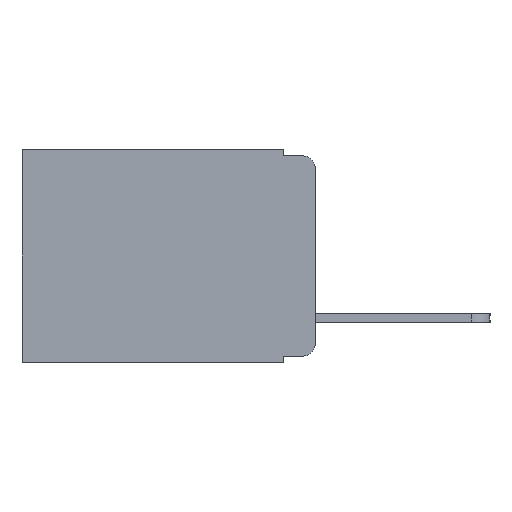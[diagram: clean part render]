
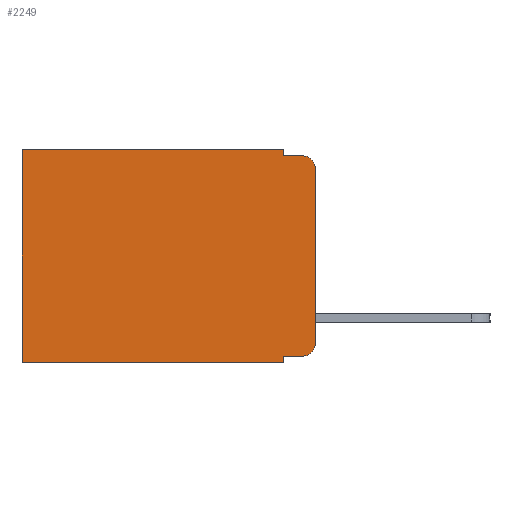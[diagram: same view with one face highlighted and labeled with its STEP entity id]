
A CAD part, left-side view. The second image highlights one B-rep face of the part: STEP entity #2249.
In plain terms, the highlighted planar face has unit normal (-1, 0, 0).
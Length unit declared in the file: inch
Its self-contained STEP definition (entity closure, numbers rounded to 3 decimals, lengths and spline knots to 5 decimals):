
#41 = CARTESIAN_POINT ( 'NONE',  ( 0.298, 0.473, 0. ) ) ;
#159 = DIRECTION ( 'NONE',  ( 0., 0., -1. ) ) ;
#184 = LINE ( 'NONE', #3766, #10985 ) ;
#445 = DIRECTION ( 'NONE',  ( 0., 1., 0. ) ) ;
#543 = ORIENTED_EDGE ( 'NONE', *, *, #4865, .F. ) ;
#1280 = CARTESIAN_POINT ( 'NONE',  ( 0.298, 0.051, -0.333 ) ) ;
#1439 = VECTOR ( 'NONE', #3045, 39.37008 ) ;
#1519 = LINE ( 'NONE', #2799, #8188 ) ;
#1610 = CARTESIAN_POINT ( 'NONE',  ( 0.298, 0.051, 0. ) ) ;
#1656 = AXIS2_PLACEMENT_3D ( 'NONE', #9635, #9394, #10530 ) ;
#1997 = ORIENTED_EDGE ( 'NONE', *, *, #7256, .F. ) ;
#2103 = CARTESIAN_POINT ( 'NONE',  ( 0.298, 0., -0.03 ) ) ;
#2249 = ADVANCED_FACE ( 'NONE', ( #2327 ), #7450, .F. ) ;
#2327 = FACE_OUTER_BOUND ( 'NONE', #2737, .T. ) ;
#2385 = VERTEX_POINT ( 'NONE', #4756 ) ;
#2593 = VERTEX_POINT ( 'NONE', #4092 ) ;
#2705 = VECTOR ( 'NONE', #5661, 39.37008 ) ;
#2737 = EDGE_LOOP ( 'NONE', ( #7662, #4558, #4544, #8062, #3162, #4737, #1997, #543, #10494, #10239 ) ) ;
#2799 = CARTESIAN_POINT ( 'NONE',  ( 0.298, 0., 0. ) ) ;
#2923 = DIRECTION ( 'NONE',  ( 0., 0., -1. ) ) ;
#2946 = CARTESIAN_POINT ( 'NONE',  ( 0.298, 0.473, 0. ) ) ;
#3045 = DIRECTION ( 'NONE',  ( 0., -1., 0. ) ) ;
#3051 = EDGE_CURVE ( 'NONE', #2385, #2593, #7707, .T. ) ;
#3162 = ORIENTED_EDGE ( 'NONE', *, *, #10858, .T. ) ;
#3249 = VECTOR ( 'NONE', #159, 39.37008 ) ;
#3407 = VECTOR ( 'NONE', #11004, 39.37008 ) ;
#3602 = AXIS2_PLACEMENT_3D ( 'NONE', #5839, #8775, #5685 ) ;
#3766 = CARTESIAN_POINT ( 'NONE',  ( 0.298, 0.051, 0. ) ) ;
#3966 = VERTEX_POINT ( 'NONE', #6133 ) ;
#3986 = VERTEX_POINT ( 'NONE', #1610 ) ;
#4092 = CARTESIAN_POINT ( 'NONE',  ( 0.298, 0., -0.313 ) ) ;
#4104 = VERTEX_POINT ( 'NONE', #2103 ) ;
#4249 = EDGE_CURVE ( 'NONE', #7365, #2385, #10185, .T. ) ;
#4544 = ORIENTED_EDGE ( 'NONE', *, *, #7107, .F. ) ;
#4558 = ORIENTED_EDGE ( 'NONE', *, *, #7637, .T. ) ;
#4737 = ORIENTED_EDGE ( 'NONE', *, *, #5451, .T. ) ;
#4756 = CARTESIAN_POINT ( 'NONE',  ( 0.298, 0.02, -0.333 ) ) ;
#4768 = CARTESIAN_POINT ( 'NONE',  ( 0.298, 0.051, -0.343 ) ) ;
#4865 = EDGE_CURVE ( 'NONE', #7365, #6795, #9928, .T. ) ;
#4984 = VERTEX_POINT ( 'NONE', #10301 ) ;
#5124 = CARTESIAN_POINT ( 'NONE',  ( 0.298, 0.02, -0.03 ) ) ;
#5451 = EDGE_CURVE ( 'NONE', #5745, #3966, #7301, .T. ) ;
#5661 = DIRECTION ( 'NONE',  ( 0., 0., -1. ) ) ;
#5685 = DIRECTION ( 'NONE',  ( 0., 0., -1. ) ) ;
#5745 = VERTEX_POINT ( 'NONE', #41 ) ;
#5839 = CARTESIAN_POINT ( 'NONE',  ( 0.298, 0., 0. ) ) ;
#5983 = DIRECTION ( 'NONE',  ( 0., 0., -1. ) ) ;
#6017 = EDGE_CURVE ( 'NONE', #3986, #4984, #184, .T. ) ;
#6046 = LINE ( 'NONE', #6265, #3407 ) ;
#6133 = CARTESIAN_POINT ( 'NONE',  ( 0.298, 0.473, -0.343 ) ) ;
#6265 = CARTESIAN_POINT ( 'NONE',  ( 0.298, 0., 0. ) ) ;
#6286 = CARTESIAN_POINT ( 'NONE',  ( 0.298, 0.051, 0. ) ) ;
#6609 = CARTESIAN_POINT ( 'NONE',  ( 0.298, 0.051, -0.333 ) ) ;
#6795 = VERTEX_POINT ( 'NONE', #4768 ) ;
#7107 = EDGE_CURVE ( 'NONE', #4984, #10355, #10242, .T. ) ;
#7256 = EDGE_CURVE ( 'NONE', #6795, #3966, #10835, .T. ) ;
#7301 = LINE ( 'NONE', #2946, #2705 ) ;
#7365 = VERTEX_POINT ( 'NONE', #1280 ) ;
#7450 = PLANE ( 'NONE',  #3602 ) ;
#7637 = EDGE_CURVE ( 'NONE', #4104, #10355, #9751, .T. ) ;
#7662 = ORIENTED_EDGE ( 'NONE', *, *, #10304, .F. ) ;
#7707 = CIRCLE ( 'NONE', #1656, 0.02 ) ;
#8061 = VECTOR ( 'NONE', #9763, 39.37008 ) ;
#8062 = ORIENTED_EDGE ( 'NONE', *, *, #6017, .F. ) ;
#8188 = VECTOR ( 'NONE', #9561, 39.37008 ) ;
#8421 = AXIS2_PLACEMENT_3D ( 'NONE', #5124, #10755, #5983 ) ;
#8756 = VECTOR ( 'NONE', #445, 39.37008 ) ;
#8775 = DIRECTION ( 'NONE',  ( 1., 0., 0. ) ) ;
#8828 = CARTESIAN_POINT ( 'NONE',  ( 0.298, 0.02, -0.01 ) ) ;
#9394 = DIRECTION ( 'NONE',  ( -1., 0., 0. ) ) ;
#9561 = DIRECTION ( 'NONE',  ( 0., 0., -1. ) ) ;
#9635 = CARTESIAN_POINT ( 'NONE',  ( 0.298, 0.02, -0.313 ) ) ;
#9725 = CARTESIAN_POINT ( 'NONE',  ( 0.298, 0., -0.343 ) ) ;
#9751 = CIRCLE ( 'NONE', #8421, 0.02 ) ;
#9763 = DIRECTION ( 'NONE',  ( 0., -1., 0. ) ) ;
#9928 = LINE ( 'NONE', #6286, #3249 ) ;
#10185 = LINE ( 'NONE', #6609, #8061 ) ;
#10239 = ORIENTED_EDGE ( 'NONE', *, *, #3051, .T. ) ;
#10242 = LINE ( 'NONE', #10575, #1439 ) ;
#10301 = CARTESIAN_POINT ( 'NONE',  ( 0.298, 0.051, -0.01 ) ) ;
#10304 = EDGE_CURVE ( 'NONE', #4104, #2593, #1519, .T. ) ;
#10355 = VERTEX_POINT ( 'NONE', #8828 ) ;
#10494 = ORIENTED_EDGE ( 'NONE', *, *, #4249, .T. ) ;
#10530 = DIRECTION ( 'NONE',  ( 0., 0., -1. ) ) ;
#10575 = CARTESIAN_POINT ( 'NONE',  ( 0.298, 0.051, -0.01 ) ) ;
#10755 = DIRECTION ( 'NONE',  ( -1., 0., 0. ) ) ;
#10835 = LINE ( 'NONE', #9725, #8756 ) ;
#10858 = EDGE_CURVE ( 'NONE', #3986, #5745, #6046, .T. ) ;
#10985 = VECTOR ( 'NONE', #2923, 39.37008 ) ;
#11004 = DIRECTION ( 'NONE',  ( 0., 1., 0. ) ) ;
